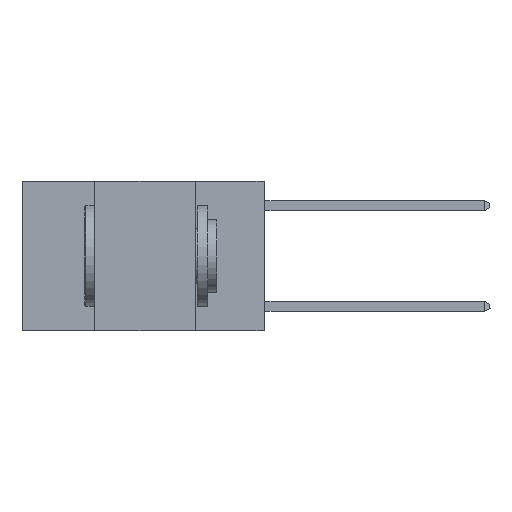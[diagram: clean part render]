
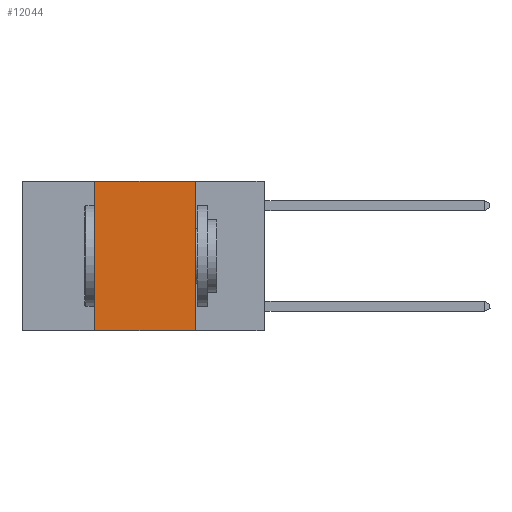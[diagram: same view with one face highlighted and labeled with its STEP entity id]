
A CAD part, left-side view. The second image highlights one B-rep face of the part: STEP entity #12044.
In plain terms, the highlighted planar face has unit normal (-1, 0, 0).
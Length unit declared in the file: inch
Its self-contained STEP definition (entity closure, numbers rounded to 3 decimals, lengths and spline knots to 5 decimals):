
#334 = ORIENTED_EDGE ( 'NONE', *, *, #3223, .F. ) ;
#434 = CARTESIAN_POINT ( 'NONE',  ( 0., 0.6, 0. ) ) ;
#598 = EDGE_LOOP ( 'NONE', ( #3942, #334, #15449, #12985 ) ) ;
#1022 = AXIS2_PLACEMENT_3D ( 'NONE', #14706, #1665, #7464 ) ;
#1242 = CARTESIAN_POINT ( 'NONE',  ( 0., 0.42, 0. ) ) ;
#1665 = DIRECTION ( 'NONE',  ( 1., 0., 0. ) ) ;
#2850 = CARTESIAN_POINT ( 'NONE',  ( 0., 0.17, -0.37 ) ) ;
#3223 = EDGE_CURVE ( 'NONE', #11329, #3674, #10535, .T. ) ;
#3478 = DIRECTION ( 'NONE',  ( 0., -1., 0. ) ) ;
#3508 = LINE ( 'NONE', #10937, #5067 ) ;
#3674 = VERTEX_POINT ( 'NONE', #10702 ) ;
#3820 = CARTESIAN_POINT ( 'NONE',  ( 0., 0.42, -0.37 ) ) ;
#3942 = ORIENTED_EDGE ( 'NONE', *, *, #5880, .F. ) ;
#4883 = PLANE ( 'NONE',  #1022 ) ;
#5067 = VECTOR ( 'NONE', #15139, 39.37008 ) ;
#5300 = LINE ( 'NONE', #6660, #16917 ) ;
#5478 = DIRECTION ( 'NONE',  ( 0., 0., -1. ) ) ;
#5880 = EDGE_CURVE ( 'NONE', #3674, #12754, #18412, .T. ) ;
#6136 = FACE_OUTER_BOUND ( 'NONE', #598, .T. ) ;
#6660 = CARTESIAN_POINT ( 'NONE',  ( 0., 0.6, -0.37 ) ) ;
#7464 = DIRECTION ( 'NONE',  ( 0., 0., -1. ) ) ;
#10535 = LINE ( 'NONE', #434, #16375 ) ;
#10702 = CARTESIAN_POINT ( 'NONE',  ( 0., 0.17, 0. ) ) ;
#10937 = CARTESIAN_POINT ( 'NONE',  ( 0., 0.42, 0. ) ) ;
#11087 = CARTESIAN_POINT ( 'NONE',  ( 0., 0.17, 0. ) ) ;
#11329 = VERTEX_POINT ( 'NONE', #1242 ) ;
#12044 = ADVANCED_FACE ( 'NONE', ( #6136 ), #4883, .F. ) ;
#12754 = VERTEX_POINT ( 'NONE', #2850 ) ;
#12985 = ORIENTED_EDGE ( 'NONE', *, *, #16719, .T. ) ;
#14706 = CARTESIAN_POINT ( 'NONE',  ( 0., 0.6, 0. ) ) ;
#15139 = DIRECTION ( 'NONE',  ( 0., 0., 1. ) ) ;
#15267 = EDGE_CURVE ( 'NONE', #16230, #11329, #3508, .T. ) ;
#15449 = ORIENTED_EDGE ( 'NONE', *, *, #15267, .F. ) ;
#16230 = VERTEX_POINT ( 'NONE', #3820 ) ;
#16375 = VECTOR ( 'NONE', #3478, 39.37008 ) ;
#16719 = EDGE_CURVE ( 'NONE', #16230, #12754, #5300, .T. ) ;
#16917 = VECTOR ( 'NONE', #18267, 39.37008 ) ;
#18267 = DIRECTION ( 'NONE',  ( 0., -1., 0. ) ) ;
#18384 = VECTOR ( 'NONE', #5478, 39.37008 ) ;
#18412 = LINE ( 'NONE', #11087, #18384 ) ;
